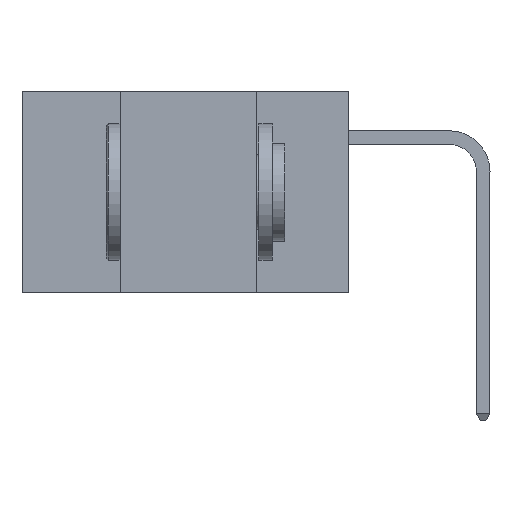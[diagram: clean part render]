
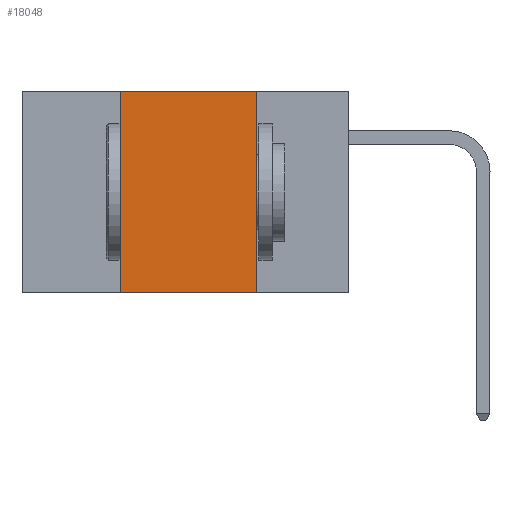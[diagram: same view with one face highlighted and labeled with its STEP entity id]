
A CAD part, left-side view. The second image highlights one B-rep face of the part: STEP entity #18048.
In plain terms, the highlighted planar face has unit normal (-1, 0, 0).
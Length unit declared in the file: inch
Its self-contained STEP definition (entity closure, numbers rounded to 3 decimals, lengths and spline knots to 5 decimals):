
#124 = EDGE_LOOP ( 'NONE', ( #4785, #33925, #36571, #20811 ) ) ;
#1239 = PLANE ( 'NONE',  #15744 ) ;
#1465 = VERTEX_POINT ( 'NONE', #3730 ) ;
#2652 = FACE_OUTER_BOUND ( 'NONE', #124, .T. ) ;
#2804 = DIRECTION ( 'NONE',  ( 0., 0., -1. ) ) ;
#3384 = DIRECTION ( 'NONE',  ( 0., -1., 0. ) ) ;
#3730 = CARTESIAN_POINT ( 'NONE',  ( 0., 0.42, -0.37 ) ) ;
#4785 = ORIENTED_EDGE ( 'NONE', *, *, #24621, .F. ) ;
#5148 = VECTOR ( 'NONE', #3384, 39.37008 ) ;
#5861 = LINE ( 'NONE', #32894, #21285 ) ;
#6867 = EDGE_CURVE ( 'NONE', #18367, #34840, #5861, .T. ) ;
#8659 = CARTESIAN_POINT ( 'NONE',  ( 0., 0.42, 0. ) ) ;
#10105 = DIRECTION ( 'NONE',  ( 1., 0., 0. ) ) ;
#12406 = VECTOR ( 'NONE', #14884, 39.37008 ) ;
#14884 = DIRECTION ( 'NONE',  ( 0., 0., 1. ) ) ;
#15224 = EDGE_CURVE ( 'NONE', #1465, #28503, #27952, .T. ) ;
#15744 = AXIS2_PLACEMENT_3D ( 'NONE', #27076, #10105, #29945 ) ;
#16856 = CARTESIAN_POINT ( 'NONE',  ( 0., 0.17, 0. ) ) ;
#17119 = EDGE_CURVE ( 'NONE', #1465, #18367, #27374, .T. ) ;
#18048 = ADVANCED_FACE ( 'NONE', ( #2652 ), #1239, .F. ) ;
#18075 = CARTESIAN_POINT ( 'NONE',  ( 0., 0.6, -0.37 ) ) ;
#18367 = VERTEX_POINT ( 'NONE', #8659 ) ;
#20811 = ORIENTED_EDGE ( 'NONE', *, *, #15224, .T. ) ;
#21285 = VECTOR ( 'NONE', #35500, 39.37008 ) ;
#22982 = CARTESIAN_POINT ( 'NONE',  ( 0., 0.17, -0.37 ) ) ;
#24621 = EDGE_CURVE ( 'NONE', #34840, #28503, #33689, .T. ) ;
#26137 = VECTOR ( 'NONE', #2804, 39.37008 ) ;
#27076 = CARTESIAN_POINT ( 'NONE',  ( 0., 0.6, 0. ) ) ;
#27374 = LINE ( 'NONE', #31754, #12406 ) ;
#27952 = LINE ( 'NONE', #18075, #5148 ) ;
#28503 = VERTEX_POINT ( 'NONE', #22982 ) ;
#29945 = DIRECTION ( 'NONE',  ( 0., 0., -1. ) ) ;
#31754 = CARTESIAN_POINT ( 'NONE',  ( 0., 0.42, 0. ) ) ;
#32894 = CARTESIAN_POINT ( 'NONE',  ( 0., 0.6, 0. ) ) ;
#33689 = LINE ( 'NONE', #37025, #26137 ) ;
#33925 = ORIENTED_EDGE ( 'NONE', *, *, #6867, .F. ) ;
#34840 = VERTEX_POINT ( 'NONE', #16856 ) ;
#35500 = DIRECTION ( 'NONE',  ( 0., -1., 0. ) ) ;
#36571 = ORIENTED_EDGE ( 'NONE', *, *, #17119, .F. ) ;
#37025 = CARTESIAN_POINT ( 'NONE',  ( 0., 0.17, 0. ) ) ;
